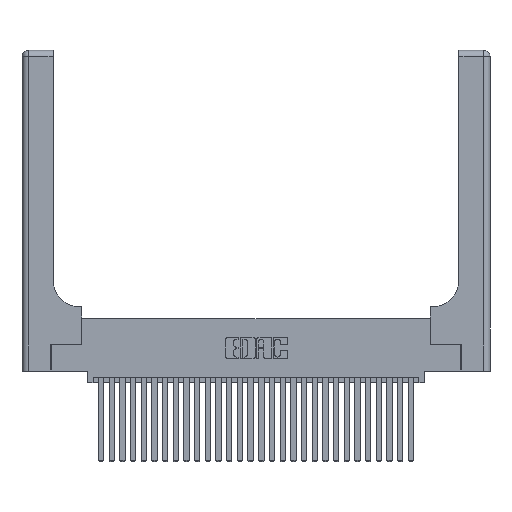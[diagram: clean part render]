
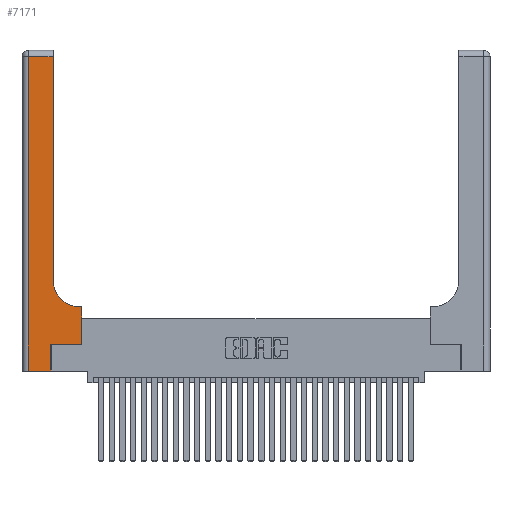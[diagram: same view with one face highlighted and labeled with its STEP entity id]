
A CAD part, top view. The second image highlights one B-rep face of the part: STEP entity #7171.
In plain terms, the highlighted planar face has unit normal (0, 0, 1).
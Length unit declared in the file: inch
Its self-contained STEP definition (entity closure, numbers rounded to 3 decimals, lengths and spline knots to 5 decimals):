
#155 = DIRECTION ( 'NONE',  ( 0., -1., 0. ) ) ;
#578 = LINE ( 'NONE', #9692, #13025 ) ;
#809 = CARTESIAN_POINT ( 'NONE',  ( 0.269, 0.25, 0.37 ) ) ;
#1455 = DIRECTION ( 'NONE',  ( 0., 0., -1. ) ) ;
#1714 = ORIENTED_EDGE ( 'NONE', *, *, #14173, .T. ) ;
#2159 = ORIENTED_EDGE ( 'NONE', *, *, #16255, .T. ) ;
#2490 = CARTESIAN_POINT ( 'NONE',  ( 0., 3., 0.37 ) ) ;
#2796 = VECTOR ( 'NONE', #15042, 39.37008 ) ;
#2923 = LINE ( 'NONE', #809, #27058 ) ;
#3031 = EDGE_CURVE ( 'NONE', #30044, #22222, #578, .T. ) ;
#3175 = DIRECTION ( 'NONE',  ( 1., 0., 0. ) ) ;
#3725 = EDGE_CURVE ( 'NONE', #25810, #30044, #6839, .T. ) ;
#4174 = LINE ( 'NONE', #21415, #15844 ) ;
#4281 = LINE ( 'NONE', #12716, #2796 ) ;
#4513 = DIRECTION ( 'NONE',  ( -1., 0., 0. ) ) ;
#5090 = DIRECTION ( 'NONE',  ( -1., 0., 0. ) ) ;
#5682 = VECTOR ( 'NONE', #4513, 39.37008 ) ;
#5922 = LINE ( 'NONE', #28196, #17595 ) ;
#6740 = VERTEX_POINT ( 'NONE', #26641 ) ;
#6839 = LINE ( 'NONE', #23596, #18513 ) ;
#7163 = AXIS2_PLACEMENT_3D ( 'NONE', #15441, #1455, #17789 ) ;
#7171 = ADVANCED_FACE ( 'NONE', ( #21200 ), #16491, .F. ) ;
#7190 = DIRECTION ( 'NONE',  ( -1., 0., 0. ) ) ;
#7415 = CARTESIAN_POINT ( 'NONE',  ( 0.5415, 0.6, 0.37 ) ) ;
#9692 = CARTESIAN_POINT ( 'NONE',  ( 0.269, 0., 0.37 ) ) ;
#10545 = CIRCLE ( 'NONE', #7163, 0.25 ) ;
#11631 = VERTEX_POINT ( 'NONE', #17509 ) ;
#11855 = LINE ( 'NONE', #20835, #5682 ) ;
#12047 = ORIENTED_EDGE ( 'NONE', *, *, #21639, .T. ) ;
#12716 = CARTESIAN_POINT ( 'NONE',  ( 0.5585, 0.25, 0.37 ) ) ;
#13025 = VECTOR ( 'NONE', #26079, 39.37008 ) ;
#13038 = VERTEX_POINT ( 'NONE', #18552 ) ;
#13144 = ORIENTED_EDGE ( 'NONE', *, *, #3031, .T. ) ;
#13341 = EDGE_CURVE ( 'NONE', #6740, #22464, #4281, .T. ) ;
#13427 = ORIENTED_EDGE ( 'NONE', *, *, #17677, .T. ) ;
#14173 = EDGE_CURVE ( 'NONE', #22464, #27997, #11855, .T. ) ;
#14582 = LINE ( 'NONE', #30182, #26333 ) ;
#15042 = DIRECTION ( 'NONE',  ( 0., 1., 0. ) ) ;
#15337 = VERTEX_POINT ( 'NONE', #17788 ) ;
#15441 = CARTESIAN_POINT ( 'NONE',  ( 0.5415, 0.85, 0.37 ) ) ;
#15474 = CARTESIAN_POINT ( 'NONE',  ( 0.269, 0., 0.37 ) ) ;
#15844 = VECTOR ( 'NONE', #5090, 39.37008 ) ;
#16187 = DIRECTION ( 'NONE',  ( 0., 1., 0. ) ) ;
#16255 = EDGE_CURVE ( 'NONE', #13038, #25810, #5922, .T. ) ;
#16491 = PLANE ( 'NONE',  #27937 ) ;
#17348 = EDGE_CURVE ( 'NONE', #11631, #15337, #14582, .T. ) ;
#17509 = CARTESIAN_POINT ( 'NONE',  ( 0.2915, 0.85, 0.37 ) ) ;
#17595 = VECTOR ( 'NONE', #155, 39.37008 ) ;
#17677 = EDGE_CURVE ( 'NONE', #27997, #11631, #10545, .T. ) ;
#17788 = CARTESIAN_POINT ( 'NONE',  ( 0.2915, 2.94, 0.37 ) ) ;
#17789 = DIRECTION ( 'NONE',  ( 1., 0., 0. ) ) ;
#17889 = ORIENTED_EDGE ( 'NONE', *, *, #3725, .T. ) ;
#18513 = VECTOR ( 'NONE', #21234, 39.37008 ) ;
#18552 = CARTESIAN_POINT ( 'NONE',  ( 0.06, 2.94, 0.37 ) ) ;
#20835 = CARTESIAN_POINT ( 'NONE',  ( 0.2915, 0.6, 0.37 ) ) ;
#21196 = DIRECTION ( 'NONE',  ( 0., 0., -1. ) ) ;
#21200 = FACE_OUTER_BOUND ( 'NONE', #25737, .T. ) ;
#21234 = DIRECTION ( 'NONE',  ( 1., 0., 0. ) ) ;
#21415 = CARTESIAN_POINT ( 'NONE',  ( 0., 2.94, 0.37 ) ) ;
#21639 = EDGE_CURVE ( 'NONE', #22222, #6740, #2923, .T. ) ;
#22222 = VERTEX_POINT ( 'NONE', #27061 ) ;
#22464 = VERTEX_POINT ( 'NONE', #25923 ) ;
#22711 = ORIENTED_EDGE ( 'NONE', *, *, #13341, .T. ) ;
#22978 = ORIENTED_EDGE ( 'NONE', *, *, #17348, .T. ) ;
#23596 = CARTESIAN_POINT ( 'NONE',  ( 0., 0., 0.37 ) ) ;
#25737 = EDGE_LOOP ( 'NONE', ( #22978, #27386, #2159, #17889, #13144, #12047, #22711, #1714, #13427 ) ) ;
#25810 = VERTEX_POINT ( 'NONE', #27477 ) ;
#25923 = CARTESIAN_POINT ( 'NONE',  ( 0.5585, 0.6, 0.37 ) ) ;
#26076 = EDGE_CURVE ( 'NONE', #15337, #13038, #4174, .T. ) ;
#26079 = DIRECTION ( 'NONE',  ( 0., 1., 0. ) ) ;
#26333 = VECTOR ( 'NONE', #16187, 39.37008 ) ;
#26641 = CARTESIAN_POINT ( 'NONE',  ( 0.5585, 0.25, 0.37 ) ) ;
#27058 = VECTOR ( 'NONE', #3175, 39.37008 ) ;
#27061 = CARTESIAN_POINT ( 'NONE',  ( 0.269, 0.25, 0.37 ) ) ;
#27386 = ORIENTED_EDGE ( 'NONE', *, *, #26076, .T. ) ;
#27477 = CARTESIAN_POINT ( 'NONE',  ( 0.06, 0., 0.37 ) ) ;
#27937 = AXIS2_PLACEMENT_3D ( 'NONE', #2490, #21196, #7190 ) ;
#27997 = VERTEX_POINT ( 'NONE', #7415 ) ;
#28196 = CARTESIAN_POINT ( 'NONE',  ( 0.06, 3., 0.37 ) ) ;
#30044 = VERTEX_POINT ( 'NONE', #15474 ) ;
#30182 = CARTESIAN_POINT ( 'NONE',  ( 0.2915, 3., 0.37 ) ) ;
